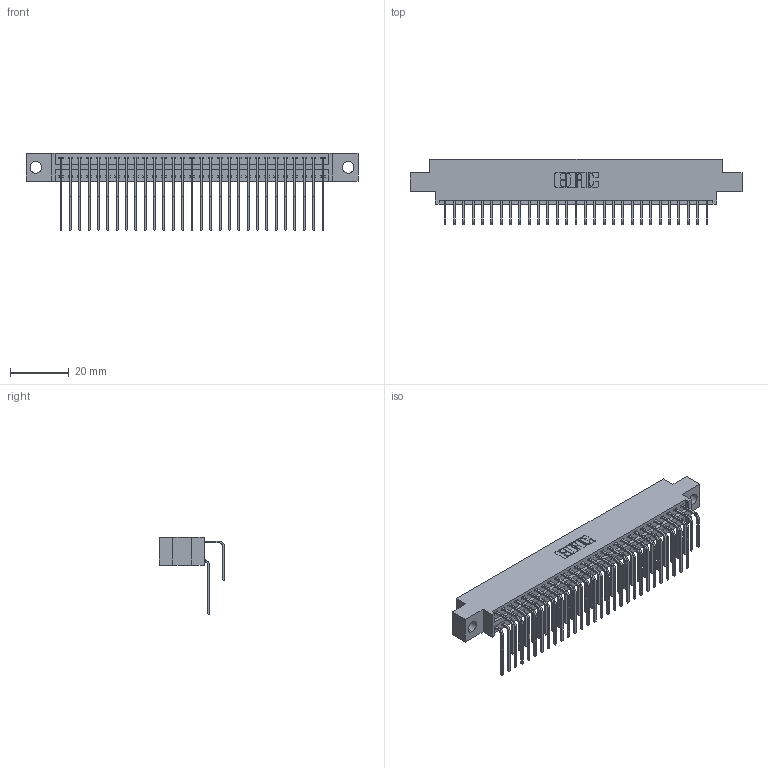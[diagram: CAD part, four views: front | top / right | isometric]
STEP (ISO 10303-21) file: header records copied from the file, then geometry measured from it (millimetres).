
FILE_DESCRIPTION (( 'STEP AP203' ), '1' );
FILE_NAME ('396-058-558-804.STEP', '2019-11-03T09:31:54', ( '' ), ( '' ), 'SwSTEP 2.0', 'SolidWorks 2016', '' );
FILE_SCHEMA (( 'CONFIG_CONTROL_DESIGN' ));
Length unit declared in the file: inch
Products named in the file (4): 345-292-001_558 559 Tail - 1; 396-058-558-804; 346 Part_0.170 Offset - 0.156 Dia-TH; 345-292-001_558 Tail - 2
Assembly tree (59 placements, depth 2):
  396-058-558-804
    346 Part_0.170 Offset - 0.156 Dia-TH
    345-292-001_558 559 Tail - 1  x29
    345-292-001_558 Tail - 2  x29
Bounding box: 112.65 x 22.16 x 26.16 mm (x, y, z)
Volume: 10975.8 mm3; surface area: 16480.8 mm2
Topology: 59 solids, 59 shells, 3258 faces, 9679 edges, 6374 vertices
Faces by surface type: plane 2226, cylinder 1032
Entity records: 22595 total; most frequent: CARTESIAN_POINT 3795, ORIENTED_EDGE 3678, DIRECTION 3367, EDGE_CURVE 1839, VECTOR 1551, LINE 1551, VERTEX_POINT 1222, AXIS2_PLACEMENT_3D 908
